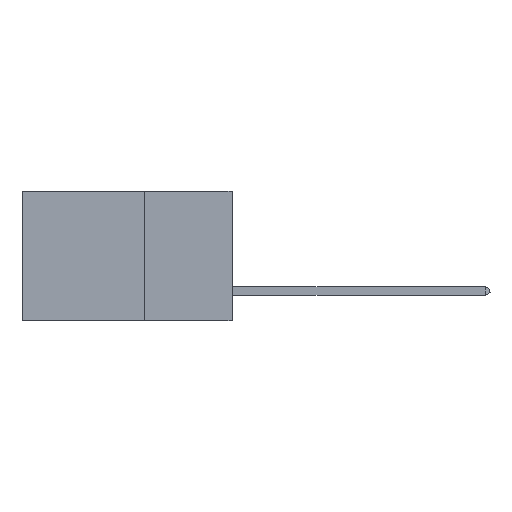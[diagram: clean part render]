
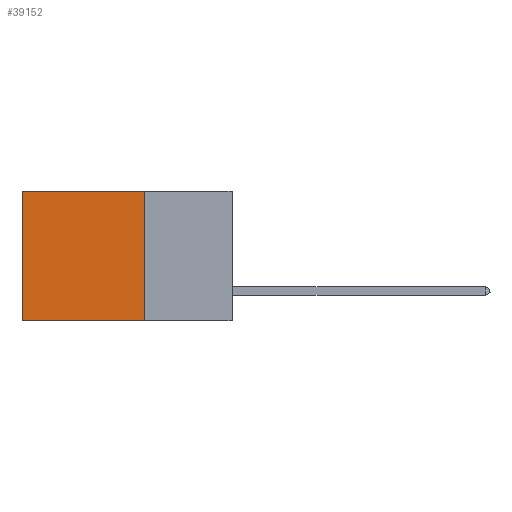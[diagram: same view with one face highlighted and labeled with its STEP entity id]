
A CAD part, left-side view. The second image highlights one B-rep face of the part: STEP entity #39152.
In plain terms, the highlighted planar face has unit normal (-1, 0, 0).
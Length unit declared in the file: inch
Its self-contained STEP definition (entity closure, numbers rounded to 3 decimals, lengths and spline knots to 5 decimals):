
#181 = DIRECTION ( 'NONE',  ( 0., 1., 0. ) ) ;
#1043 = EDGE_CURVE ( 'NONE', #24309, #36082, #6331, .T. ) ;
#1948 = VERTEX_POINT ( 'NONE', #5469 ) ;
#2082 = LINE ( 'NONE', #38077, #18444 ) ;
#2379 = EDGE_CURVE ( 'NONE', #32721, #1948, #15408, .T. ) ;
#2947 = CARTESIAN_POINT ( 'NONE',  ( 0.2875, 0.6, -0.37 ) ) ;
#3113 = EDGE_LOOP ( 'NONE', ( #21519, #10375, #43336, #6005 ) ) ;
#3775 = DIRECTION ( 'NONE',  ( 1., 0., 0. ) ) ;
#5469 = CARTESIAN_POINT ( 'NONE',  ( 0.2875, 0.6, 0. ) ) ;
#6005 = ORIENTED_EDGE ( 'NONE', *, *, #2379, .T. ) ;
#6331 = LINE ( 'NONE', #23486, #26445 ) ;
#9962 = VECTOR ( 'NONE', #12652, 39.37008 ) ;
#10375 = ORIENTED_EDGE ( 'NONE', *, *, #1043, .F. ) ;
#11630 = CARTESIAN_POINT ( 'NONE',  ( 0.2875, 0.25, 0. ) ) ;
#12652 = DIRECTION ( 'NONE',  ( 0., 0., -1. ) ) ;
#15109 = AXIS2_PLACEMENT_3D ( 'NONE', #39116, #3775, #38962 ) ;
#15408 = LINE ( 'NONE', #39379, #28473 ) ;
#17015 = LINE ( 'NONE', #36568, #9962 ) ;
#18444 = VECTOR ( 'NONE', #44931, 39.37008 ) ;
#21519 = ORIENTED_EDGE ( 'NONE', *, *, #28451, .T. ) ;
#22630 = FACE_OUTER_BOUND ( 'NONE', #3113, .T. ) ;
#23486 = CARTESIAN_POINT ( 'NONE',  ( 0.2875, 0.25, -0.37 ) ) ;
#24309 = VERTEX_POINT ( 'NONE', #32486 ) ;
#26445 = VECTOR ( 'NONE', #181, 39.37008 ) ;
#28451 = EDGE_CURVE ( 'NONE', #1948, #36082, #17015, .T. ) ;
#28473 = VECTOR ( 'NONE', #35543, 39.37008 ) ;
#30433 = EDGE_CURVE ( 'NONE', #32721, #24309, #2082, .T. ) ;
#32486 = CARTESIAN_POINT ( 'NONE',  ( 0.2875, 0.25, -0.37 ) ) ;
#32721 = VERTEX_POINT ( 'NONE', #11630 ) ;
#35434 = PLANE ( 'NONE',  #15109 ) ;
#35543 = DIRECTION ( 'NONE',  ( 0., 1., 0. ) ) ;
#36082 = VERTEX_POINT ( 'NONE', #2947 ) ;
#36568 = CARTESIAN_POINT ( 'NONE',  ( 0.2875, 0.6, 0. ) ) ;
#38077 = CARTESIAN_POINT ( 'NONE',  ( 0.2875, 0.25, 0. ) ) ;
#38962 = DIRECTION ( 'NONE',  ( 0., 0., -1. ) ) ;
#39116 = CARTESIAN_POINT ( 'NONE',  ( 0.2875, 0.25, 0. ) ) ;
#39152 = ADVANCED_FACE ( 'NONE', ( #22630 ), #35434, .F. ) ;
#39379 = CARTESIAN_POINT ( 'NONE',  ( 0.2875, 0.25, 0. ) ) ;
#43336 = ORIENTED_EDGE ( 'NONE', *, *, #30433, .F. ) ;
#44931 = DIRECTION ( 'NONE',  ( 0., 0., -1. ) ) ;
